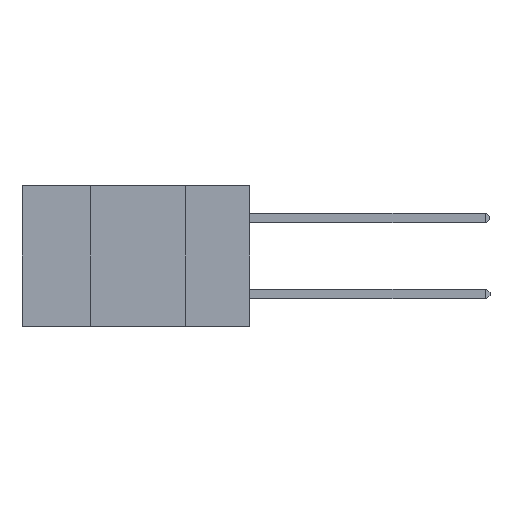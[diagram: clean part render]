
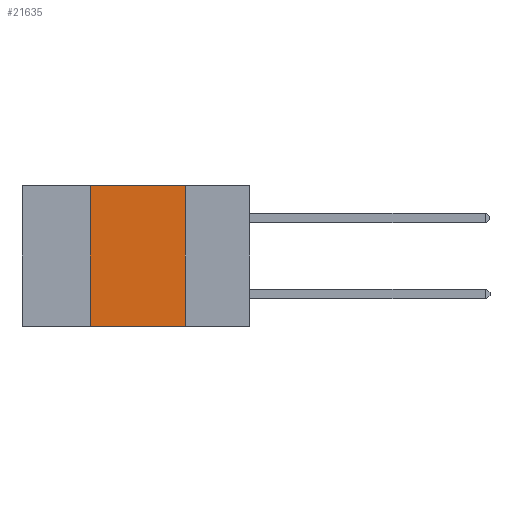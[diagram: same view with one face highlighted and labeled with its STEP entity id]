
A CAD part, left-side view. The second image highlights one B-rep face of the part: STEP entity #21635.
In plain terms, the highlighted planar face has unit normal (-1, 0, 0).
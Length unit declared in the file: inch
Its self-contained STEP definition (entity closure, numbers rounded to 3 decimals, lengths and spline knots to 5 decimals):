
#701 = DIRECTION ( 'NONE',  ( 0., 0., 1. ) ) ;
#1384 = CARTESIAN_POINT ( 'NONE',  ( 0., 0.17, 0. ) ) ;
#1538 = VERTEX_POINT ( 'NONE', #1384 ) ;
#2313 = VERTEX_POINT ( 'NONE', #11993 ) ;
#4373 = EDGE_CURVE ( 'NONE', #1538, #17559, #5006, .T. ) ;
#4477 = VECTOR ( 'NONE', #17341, 39.37008 ) ;
#4586 = DIRECTION ( 'NONE',  ( 0., -1., 0. ) ) ;
#5006 = LINE ( 'NONE', #12196, #4477 ) ;
#5128 = CARTESIAN_POINT ( 'NONE',  ( 0., 0.42, -0.37 ) ) ;
#5637 = LINE ( 'NONE', #19773, #18755 ) ;
#7353 = LINE ( 'NONE', #17711, #7863 ) ;
#7431 = FACE_OUTER_BOUND ( 'NONE', #21546, .T. ) ;
#7863 = VECTOR ( 'NONE', #701, 39.37008 ) ;
#9606 = CARTESIAN_POINT ( 'NONE',  ( 0., 0.6, 0. ) ) ;
#9798 = DIRECTION ( 'NONE',  ( 1., 0., 0. ) ) ;
#10031 = ORIENTED_EDGE ( 'NONE', *, *, #18326, .F. ) ;
#10695 = ORIENTED_EDGE ( 'NONE', *, *, #4373, .F. ) ;
#10942 = ORIENTED_EDGE ( 'NONE', *, *, #13607, .F. ) ;
#11267 = ORIENTED_EDGE ( 'NONE', *, *, #21524, .T. ) ;
#11993 = CARTESIAN_POINT ( 'NONE',  ( 0., 0.42, 0. ) ) ;
#12196 = CARTESIAN_POINT ( 'NONE',  ( 0., 0.17, 0. ) ) ;
#12293 = VECTOR ( 'NONE', #4586, 39.37008 ) ;
#13237 = CARTESIAN_POINT ( 'NONE',  ( 0., 0.6, 0. ) ) ;
#13403 = AXIS2_PLACEMENT_3D ( 'NONE', #13237, #9798, #21750 ) ;
#13607 = EDGE_CURVE ( 'NONE', #17387, #2313, #7353, .T. ) ;
#17341 = DIRECTION ( 'NONE',  ( 0., 0., -1. ) ) ;
#17387 = VERTEX_POINT ( 'NONE', #5128 ) ;
#17559 = VERTEX_POINT ( 'NONE', #20948 ) ;
#17711 = CARTESIAN_POINT ( 'NONE',  ( 0., 0.42, 0. ) ) ;
#18326 = EDGE_CURVE ( 'NONE', #2313, #1538, #21319, .T. ) ;
#18755 = VECTOR ( 'NONE', #21457, 39.37008 ) ;
#19773 = CARTESIAN_POINT ( 'NONE',  ( 0., 0.6, -0.37 ) ) ;
#20056 = PLANE ( 'NONE',  #13403 ) ;
#20948 = CARTESIAN_POINT ( 'NONE',  ( 0., 0.17, -0.37 ) ) ;
#21319 = LINE ( 'NONE', #9606, #12293 ) ;
#21457 = DIRECTION ( 'NONE',  ( 0., -1., 0. ) ) ;
#21524 = EDGE_CURVE ( 'NONE', #17387, #17559, #5637, .T. ) ;
#21546 = EDGE_LOOP ( 'NONE', ( #10695, #10031, #10942, #11267 ) ) ;
#21635 = ADVANCED_FACE ( 'NONE', ( #7431 ), #20056, .F. ) ;
#21750 = DIRECTION ( 'NONE',  ( 0., 0., -1. ) ) ;
